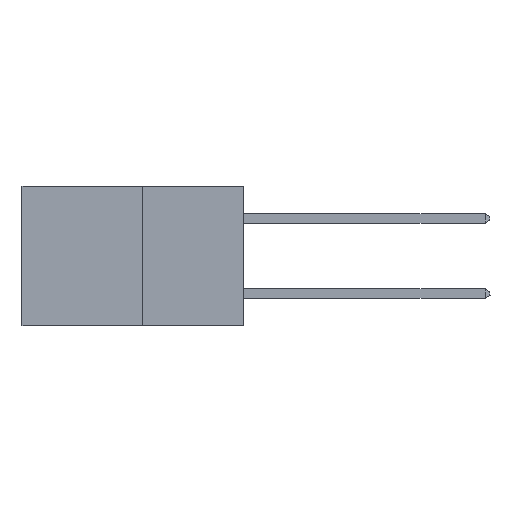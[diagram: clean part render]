
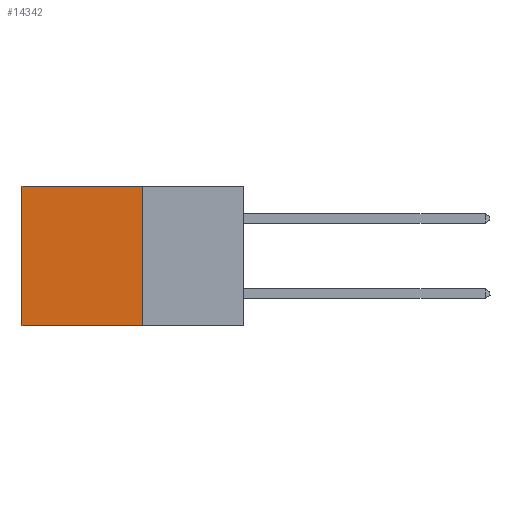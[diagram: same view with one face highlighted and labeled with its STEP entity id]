
A CAD part, left-side view. The second image highlights one B-rep face of the part: STEP entity #14342.
In plain terms, the highlighted planar face has unit normal (-1, 0, 0).
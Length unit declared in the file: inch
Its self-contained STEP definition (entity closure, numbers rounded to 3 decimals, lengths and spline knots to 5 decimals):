
#546 = VERTEX_POINT ( 'NONE', #15562 ) ;
#1808 = DIRECTION ( 'NONE',  ( 0., 0., -1. ) ) ;
#2872 = CARTESIAN_POINT ( 'NONE',  ( 0.277, 0.27, -0.37 ) ) ;
#5803 = LINE ( 'NONE', #33973, #33493 ) ;
#6203 = ORIENTED_EDGE ( 'NONE', *, *, #8457, .F. ) ;
#8457 = EDGE_CURVE ( 'NONE', #18971, #546, #27552, .T. ) ;
#9077 = VERTEX_POINT ( 'NONE', #30178 ) ;
#9191 = ORIENTED_EDGE ( 'NONE', *, *, #30006, .F. ) ;
#9485 = ORIENTED_EDGE ( 'NONE', *, *, #23341, .T. ) ;
#11740 = ORIENTED_EDGE ( 'NONE', *, *, #12125, .T. ) ;
#12023 = CARTESIAN_POINT ( 'NONE',  ( 0.277, 0.27, 0. ) ) ;
#12125 = EDGE_CURVE ( 'NONE', #32227, #9077, #24664, .T. ) ;
#12287 = VECTOR ( 'NONE', #13773, 39.37008 ) ;
#12689 = DIRECTION ( 'NONE',  ( 0., 0., -1. ) ) ;
#12713 = AXIS2_PLACEMENT_3D ( 'NONE', #29005, #34225, #18312 ) ;
#12953 = CARTESIAN_POINT ( 'NONE',  ( 0.277, 0.27, -0.37 ) ) ;
#13773 = DIRECTION ( 'NONE',  ( 0., 1., 0. ) ) ;
#14342 = ADVANCED_FACE ( 'NONE', ( #18612 ), #23676, .F. ) ;
#15562 = CARTESIAN_POINT ( 'NONE',  ( 0.277, 0.59, -0.37 ) ) ;
#16727 = EDGE_LOOP ( 'NONE', ( #9485, #6203, #9191, #11740 ) ) ;
#17104 = LINE ( 'NONE', #26215, #24337 ) ;
#18312 = DIRECTION ( 'NONE',  ( 0., 0., -1. ) ) ;
#18612 = FACE_OUTER_BOUND ( 'NONE', #16727, .T. ) ;
#18971 = VERTEX_POINT ( 'NONE', #12953 ) ;
#23341 = EDGE_CURVE ( 'NONE', #9077, #546, #5803, .T. ) ;
#23676 = PLANE ( 'NONE',  #12713 ) ;
#24337 = VECTOR ( 'NONE', #12689, 39.37008 ) ;
#24664 = LINE ( 'NONE', #12023, #30836 ) ;
#26215 = CARTESIAN_POINT ( 'NONE',  ( 0.277, 0.27, -0.37 ) ) ;
#27552 = LINE ( 'NONE', #2872, #12287 ) ;
#28475 = CARTESIAN_POINT ( 'NONE',  ( 0.277, 0.27, 0. ) ) ;
#29005 = CARTESIAN_POINT ( 'NONE',  ( 0.277, 0.27, -0.37 ) ) ;
#30006 = EDGE_CURVE ( 'NONE', #32227, #18971, #17104, .T. ) ;
#30178 = CARTESIAN_POINT ( 'NONE',  ( 0.277, 0.59, 0. ) ) ;
#30836 = VECTOR ( 'NONE', #33417, 39.37008 ) ;
#32227 = VERTEX_POINT ( 'NONE', #28475 ) ;
#33417 = DIRECTION ( 'NONE',  ( 0., 1., 0. ) ) ;
#33493 = VECTOR ( 'NONE', #1808, 39.37008 ) ;
#33973 = CARTESIAN_POINT ( 'NONE',  ( 0.277, 0.59, -0.37 ) ) ;
#34225 = DIRECTION ( 'NONE',  ( 1., 0., 0. ) ) ;
